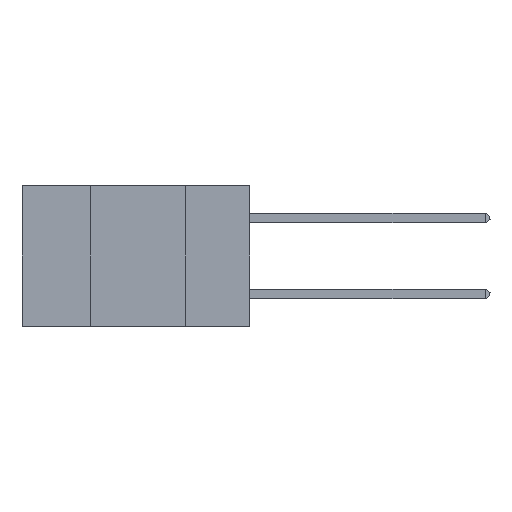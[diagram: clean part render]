
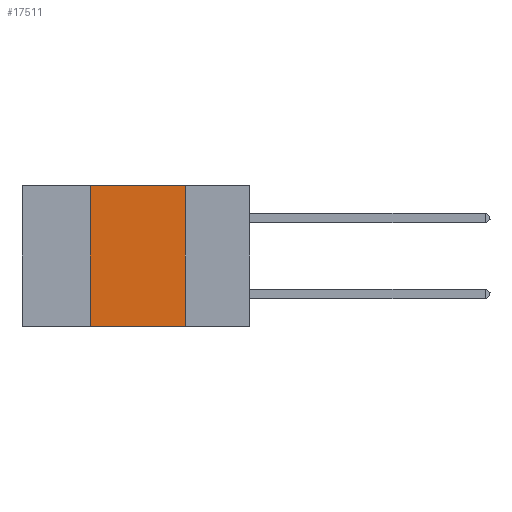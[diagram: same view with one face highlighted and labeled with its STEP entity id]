
A CAD part, left-side view. The second image highlights one B-rep face of the part: STEP entity #17511.
In plain terms, the highlighted planar face has unit normal (-1, 0, 0).
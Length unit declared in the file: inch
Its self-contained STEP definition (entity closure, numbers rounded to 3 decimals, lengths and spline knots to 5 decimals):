
#384 = DIRECTION ( 'NONE',  ( 1., 0., 0. ) ) ;
#1313 = CARTESIAN_POINT ( 'NONE',  ( 0., 0.17, 0. ) ) ;
#1362 = VECTOR ( 'NONE', #30620, 39.37008 ) ;
#2099 = VERTEX_POINT ( 'NONE', #25773 ) ;
#2367 = DIRECTION ( 'NONE',  ( 0., -1., 0. ) ) ;
#2443 = EDGE_CURVE ( 'NONE', #8430, #2099, #28675, .T. ) ;
#2538 = ORIENTED_EDGE ( 'NONE', *, *, #18058, .T. ) ;
#3225 = CARTESIAN_POINT ( 'NONE',  ( 0., 0.17, -0.37 ) ) ;
#4463 = FACE_OUTER_BOUND ( 'NONE', #5240, .T. ) ;
#4820 = ORIENTED_EDGE ( 'NONE', *, *, #25991, .F. ) ;
#5240 = EDGE_LOOP ( 'NONE', ( #9127, #9410, #4820, #2538 ) ) ;
#6306 = CARTESIAN_POINT ( 'NONE',  ( 0., 0.42, 0. ) ) ;
#7299 = VERTEX_POINT ( 'NONE', #19148 ) ;
#8430 = VERTEX_POINT ( 'NONE', #18114 ) ;
#9127 = ORIENTED_EDGE ( 'NONE', *, *, #16470, .F. ) ;
#9410 = ORIENTED_EDGE ( 'NONE', *, *, #2443, .F. ) ;
#10307 = PLANE ( 'NONE',  #26281 ) ;
#14813 = CARTESIAN_POINT ( 'NONE',  ( 0., 0.6, 0. ) ) ;
#15316 = CARTESIAN_POINT ( 'NONE',  ( 0., 0.6, 0. ) ) ;
#16470 = EDGE_CURVE ( 'NONE', #2099, #23406, #26780, .T. ) ;
#17511 = ADVANCED_FACE ( 'NONE', ( #4463 ), #10307, .F. ) ;
#17777 = DIRECTION ( 'NONE',  ( 0., 0., -1. ) ) ;
#18058 = EDGE_CURVE ( 'NONE', #7299, #23406, #25203, .T. ) ;
#18114 = CARTESIAN_POINT ( 'NONE',  ( 0., 0.42, 0. ) ) ;
#19148 = CARTESIAN_POINT ( 'NONE',  ( 0., 0.42, -0.37 ) ) ;
#21079 = VECTOR ( 'NONE', #26954, 39.37008 ) ;
#21157 = LINE ( 'NONE', #6306, #1362 ) ;
#22115 = CARTESIAN_POINT ( 'NONE',  ( 0., 0.6, -0.37 ) ) ;
#22292 = VECTOR ( 'NONE', #2367, 39.37008 ) ;
#23406 = VERTEX_POINT ( 'NONE', #3225 ) ;
#25203 = LINE ( 'NONE', #22115, #21079 ) ;
#25773 = CARTESIAN_POINT ( 'NONE',  ( 0., 0.17, 0. ) ) ;
#25991 = EDGE_CURVE ( 'NONE', #7299, #8430, #21157, .T. ) ;
#26025 = VECTOR ( 'NONE', #28498, 39.37008 ) ;
#26281 = AXIS2_PLACEMENT_3D ( 'NONE', #15316, #384, #17777 ) ;
#26780 = LINE ( 'NONE', #1313, #26025 ) ;
#26954 = DIRECTION ( 'NONE',  ( 0., -1., 0. ) ) ;
#28498 = DIRECTION ( 'NONE',  ( 0., 0., -1. ) ) ;
#28675 = LINE ( 'NONE', #14813, #22292 ) ;
#30620 = DIRECTION ( 'NONE',  ( 0., 0., 1. ) ) ;
